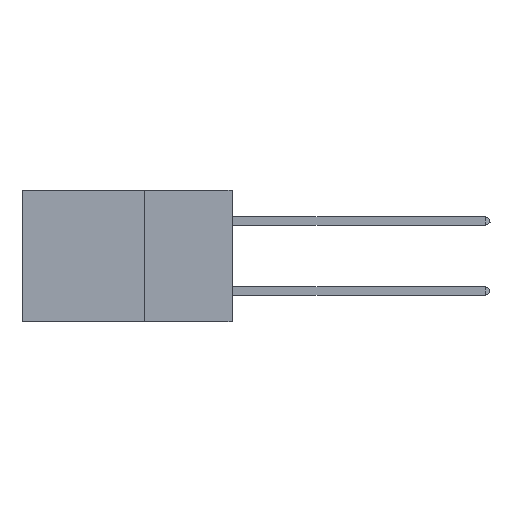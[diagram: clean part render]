
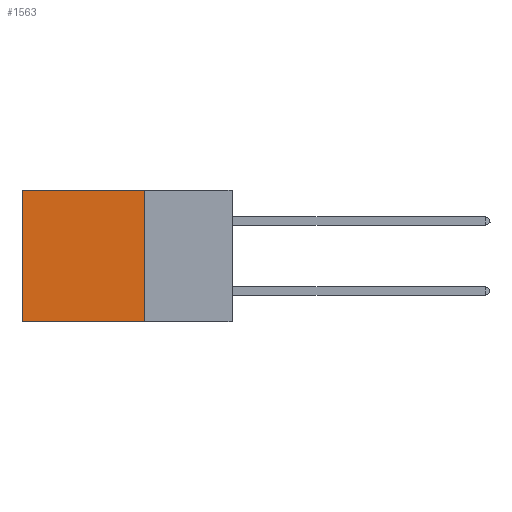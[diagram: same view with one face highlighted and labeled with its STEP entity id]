
A CAD part, left-side view. The second image highlights one B-rep face of the part: STEP entity #1563.
In plain terms, the highlighted planar face has unit normal (-1, 0, 0).
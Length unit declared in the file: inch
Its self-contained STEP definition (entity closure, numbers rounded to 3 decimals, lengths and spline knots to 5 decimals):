
#206 = CARTESIAN_POINT ( 'NONE',  ( 0.2875, 0.25, 0. ) ) ;
#370 = FACE_OUTER_BOUND ( 'NONE', #2162, .T. ) ;
#686 = LINE ( 'NONE', #2635, #6634 ) ;
#885 = AXIS2_PLACEMENT_3D ( 'NONE', #5764, #5827, #6817 ) ;
#1084 = VERTEX_POINT ( 'NONE', #4278 ) ;
#1354 = CARTESIAN_POINT ( 'NONE',  ( 0.2875, 0.6, -0.375 ) ) ;
#1563 = ADVANCED_FACE ( 'NONE', ( #370 ), #6669, .F. ) ;
#1596 = CARTESIAN_POINT ( 'NONE',  ( 0.2875, 0.25, -0.375 ) ) ;
#2162 = EDGE_LOOP ( 'NONE', ( #7489, #4806, #9333, #5802 ) ) ;
#2367 = VERTEX_POINT ( 'NONE', #206 ) ;
#2635 = CARTESIAN_POINT ( 'NONE',  ( 0.2875, 0.25, -0.375 ) ) ;
#2904 = VECTOR ( 'NONE', #5956, 39.37008 ) ;
#3236 = EDGE_CURVE ( 'NONE', #3685, #1084, #9829, .T. ) ;
#3239 = VECTOR ( 'NONE', #3284, 39.37008 ) ;
#3284 = DIRECTION ( 'NONE',  ( 0., 1., 0. ) ) ;
#3685 = VERTEX_POINT ( 'NONE', #4589 ) ;
#4278 = CARTESIAN_POINT ( 'NONE',  ( 0.2875, 0.6, -0.375 ) ) ;
#4589 = CARTESIAN_POINT ( 'NONE',  ( 0.2875, 0.6, 0. ) ) ;
#4806 = ORIENTED_EDGE ( 'NONE', *, *, #8038, .F. ) ;
#5745 = DIRECTION ( 'NONE',  ( 0., 0., -1. ) ) ;
#5764 = CARTESIAN_POINT ( 'NONE',  ( 0.2875, 0.25, -0.375 ) ) ;
#5802 = ORIENTED_EDGE ( 'NONE', *, *, #11216, .T. ) ;
#5827 = DIRECTION ( 'NONE',  ( 1., 0., 0. ) ) ;
#5956 = DIRECTION ( 'NONE',  ( 0., 1., 0. ) ) ;
#5971 = VERTEX_POINT ( 'NONE', #10775 ) ;
#6347 = LINE ( 'NONE', #11497, #3239 ) ;
#6478 = VECTOR ( 'NONE', #8858, 39.37008 ) ;
#6634 = VECTOR ( 'NONE', #5745, 39.37008 ) ;
#6669 = PLANE ( 'NONE',  #885 ) ;
#6680 = EDGE_CURVE ( 'NONE', #2367, #5971, #686, .T. ) ;
#6817 = DIRECTION ( 'NONE',  ( 0., 0., -1. ) ) ;
#7489 = ORIENTED_EDGE ( 'NONE', *, *, #3236, .T. ) ;
#8038 = EDGE_CURVE ( 'NONE', #5971, #1084, #11107, .T. ) ;
#8858 = DIRECTION ( 'NONE',  ( 0., 0., -1. ) ) ;
#9333 = ORIENTED_EDGE ( 'NONE', *, *, #6680, .F. ) ;
#9829 = LINE ( 'NONE', #1354, #6478 ) ;
#10775 = CARTESIAN_POINT ( 'NONE',  ( 0.2875, 0.25, -0.375 ) ) ;
#11107 = LINE ( 'NONE', #1596, #2904 ) ;
#11216 = EDGE_CURVE ( 'NONE', #2367, #3685, #6347, .T. ) ;
#11497 = CARTESIAN_POINT ( 'NONE',  ( 0.2875, 0.25, 0. ) ) ;
